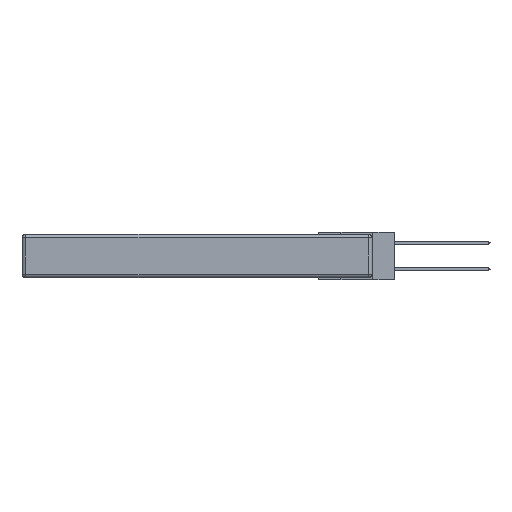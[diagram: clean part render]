
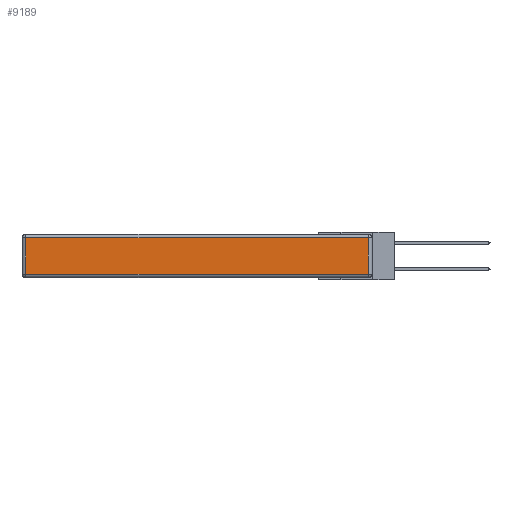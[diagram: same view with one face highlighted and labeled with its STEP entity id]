
A CAD part, left-side view. The second image highlights one B-rep face of the part: STEP entity #9189.
In plain terms, the highlighted planar face has unit normal (-1, 0, 0).
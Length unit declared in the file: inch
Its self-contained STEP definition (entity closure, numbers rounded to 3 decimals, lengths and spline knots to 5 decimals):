
#343 = ORIENTED_EDGE ( 'NONE', *, *, #18735, .T. ) ;
#1337 = CARTESIAN_POINT ( 'NONE',  ( 0., 0.03, -0.03 ) ) ;
#1487 = FACE_OUTER_BOUND ( 'NONE', #7986, .T. ) ;
#2060 = EDGE_CURVE ( 'NONE', #9943, #15534, #20413, .T. ) ;
#2188 = CARTESIAN_POINT ( 'NONE',  ( 0., 0.03, -0.343 ) ) ;
#3368 = DIRECTION ( 'NONE',  ( 0., -1., 0. ) ) ;
#3465 = CARTESIAN_POINT ( 'NONE',  ( 0., 0., -0.313 ) ) ;
#3596 = LINE ( 'NONE', #3465, #19663 ) ;
#4391 = DIRECTION ( 'NONE',  ( 0., 0., 1. ) ) ;
#4409 = CARTESIAN_POINT ( 'NONE',  ( 0., 2.72, -0.313 ) ) ;
#4613 = ORIENTED_EDGE ( 'NONE', *, *, #26358, .T. ) ;
#5014 = ORIENTED_EDGE ( 'NONE', *, *, #12182, .T. ) ;
#5989 = PLANE ( 'NONE',  #15400 ) ;
#6107 = VECTOR ( 'NONE', #9919, 39.37008 ) ;
#6226 = VERTEX_POINT ( 'NONE', #26972 ) ;
#6579 = CARTESIAN_POINT ( 'NONE',  ( 0., 2.72, -0.03 ) ) ;
#7119 = VECTOR ( 'NONE', #23177, 39.37008 ) ;
#7547 = CARTESIAN_POINT ( 'NONE',  ( 0., 2.75, -0.03 ) ) ;
#7986 = EDGE_LOOP ( 'NONE', ( #5014, #343, #23689, #4613 ) ) ;
#9189 = ADVANCED_FACE ( 'NONE', ( #1487 ), #5989, .T. ) ;
#9887 = LINE ( 'NONE', #2188, #25879 ) ;
#9919 = DIRECTION ( 'NONE',  ( 0., 1., 0. ) ) ;
#9943 = VERTEX_POINT ( 'NONE', #1337 ) ;
#12182 = EDGE_CURVE ( 'NONE', #16045, #6226, #3596, .T. ) ;
#14824 = LINE ( 'NONE', #18488, #7119 ) ;
#15400 = AXIS2_PLACEMENT_3D ( 'NONE', #21697, #23920, #26171 ) ;
#15534 = VERTEX_POINT ( 'NONE', #6579 ) ;
#16045 = VERTEX_POINT ( 'NONE', #4409 ) ;
#18488 = CARTESIAN_POINT ( 'NONE',  ( 0., 2.72, -0.343 ) ) ;
#18735 = EDGE_CURVE ( 'NONE', #6226, #9943, #9887, .T. ) ;
#19663 = VECTOR ( 'NONE', #3368, 39.37008 ) ;
#20413 = LINE ( 'NONE', #7547, #6107 ) ;
#21697 = CARTESIAN_POINT ( 'NONE',  ( 0., 0., -0.343 ) ) ;
#23177 = DIRECTION ( 'NONE',  ( 0., 0., -1. ) ) ;
#23689 = ORIENTED_EDGE ( 'NONE', *, *, #2060, .T. ) ;
#23920 = DIRECTION ( 'NONE',  ( -1., 0., 0. ) ) ;
#25879 = VECTOR ( 'NONE', #4391, 39.37008 ) ;
#26171 = DIRECTION ( 'NONE',  ( 0., 0., 1. ) ) ;
#26358 = EDGE_CURVE ( 'NONE', #15534, #16045, #14824, .T. ) ;
#26972 = CARTESIAN_POINT ( 'NONE',  ( 0., 0.03, -0.313 ) ) ;
